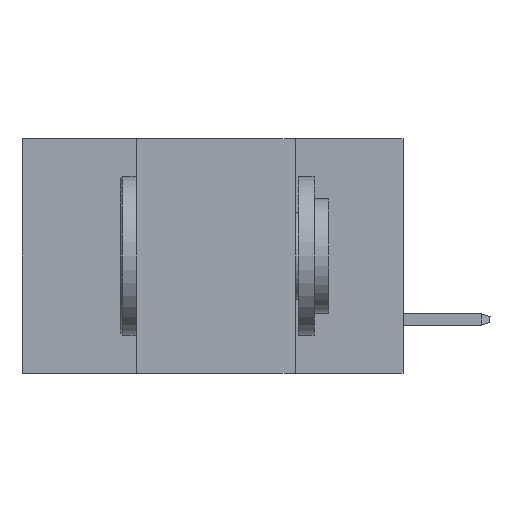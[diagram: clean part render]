
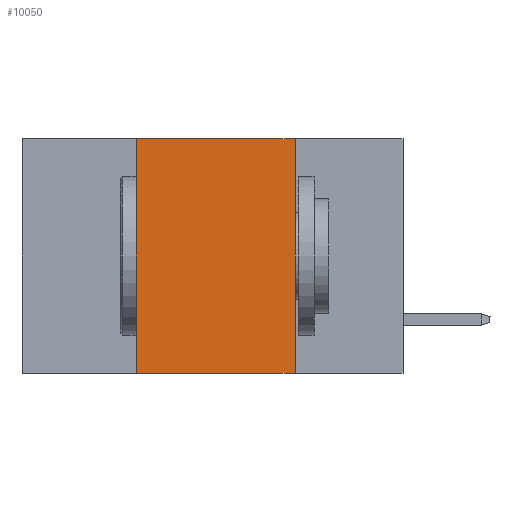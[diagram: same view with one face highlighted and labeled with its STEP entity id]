
A CAD part, left-side view. The second image highlights one B-rep face of the part: STEP entity #10050.
In plain terms, the highlighted planar face has unit normal (-1, 0, 0).
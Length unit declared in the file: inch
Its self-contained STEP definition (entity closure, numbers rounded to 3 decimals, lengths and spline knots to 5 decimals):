
#523 = DIRECTION ( 'NONE',  ( 0., 0., -1. ) ) ;
#739 = CARTESIAN_POINT ( 'NONE',  ( 0., 0.42, 0. ) ) ;
#1056 = EDGE_CURVE ( 'NONE', #2127, #8038, #10041, .T. ) ;
#1187 = VECTOR ( 'NONE', #8255, 39.37008 ) ;
#1262 = LINE ( 'NONE', #2321, #8145 ) ;
#1457 = DIRECTION ( 'NONE',  ( 1., 0., 0. ) ) ;
#1476 = LINE ( 'NONE', #10337, #1187 ) ;
#1566 = VERTEX_POINT ( 'NONE', #9105 ) ;
#1643 = VECTOR ( 'NONE', #5273, 39.37008 ) ;
#2127 = VERTEX_POINT ( 'NONE', #11695 ) ;
#2321 = CARTESIAN_POINT ( 'NONE',  ( 0., 0.17, 0. ) ) ;
#2370 = ORIENTED_EDGE ( 'NONE', *, *, #9749, .T. ) ;
#2442 = VECTOR ( 'NONE', #5596, 39.37008 ) ;
#4346 = EDGE_LOOP ( 'NONE', ( #4547, #14146, #5589, #2370 ) ) ;
#4459 = CARTESIAN_POINT ( 'NONE',  ( 0., 0.6, 0. ) ) ;
#4547 = ORIENTED_EDGE ( 'NONE', *, *, #14999, .F. ) ;
#5273 = DIRECTION ( 'NONE',  ( 0., 0., 1. ) ) ;
#5589 = ORIENTED_EDGE ( 'NONE', *, *, #1056, .F. ) ;
#5596 = DIRECTION ( 'NONE',  ( 0., -1., 0. ) ) ;
#6358 = PLANE ( 'NONE',  #14204 ) ;
#6806 = CARTESIAN_POINT ( 'NONE',  ( 0., 0.17, -0.37 ) ) ;
#8038 = VERTEX_POINT ( 'NONE', #739 ) ;
#8145 = VECTOR ( 'NONE', #13152, 39.37008 ) ;
#8255 = DIRECTION ( 'NONE',  ( 0., -1., 0. ) ) ;
#9105 = CARTESIAN_POINT ( 'NONE',  ( 0., 0.17, 0. ) ) ;
#9484 = VERTEX_POINT ( 'NONE', #6806 ) ;
#9749 = EDGE_CURVE ( 'NONE', #2127, #9484, #1476, .T. ) ;
#10041 = LINE ( 'NONE', #10121, #1643 ) ;
#10050 = ADVANCED_FACE ( 'NONE', ( #10751 ), #6358, .F. ) ;
#10121 = CARTESIAN_POINT ( 'NONE',  ( 0., 0.42, 0. ) ) ;
#10337 = CARTESIAN_POINT ( 'NONE',  ( 0., 0.6, -0.37 ) ) ;
#10751 = FACE_OUTER_BOUND ( 'NONE', #4346, .T. ) ;
#11063 = EDGE_CURVE ( 'NONE', #8038, #1566, #13765, .T. ) ;
#11695 = CARTESIAN_POINT ( 'NONE',  ( 0., 0.42, -0.37 ) ) ;
#13152 = DIRECTION ( 'NONE',  ( 0., 0., -1. ) ) ;
#13431 = CARTESIAN_POINT ( 'NONE',  ( 0., 0.6, 0. ) ) ;
#13765 = LINE ( 'NONE', #4459, #2442 ) ;
#14146 = ORIENTED_EDGE ( 'NONE', *, *, #11063, .F. ) ;
#14204 = AXIS2_PLACEMENT_3D ( 'NONE', #13431, #1457, #523 ) ;
#14999 = EDGE_CURVE ( 'NONE', #1566, #9484, #1262, .T. ) ;
